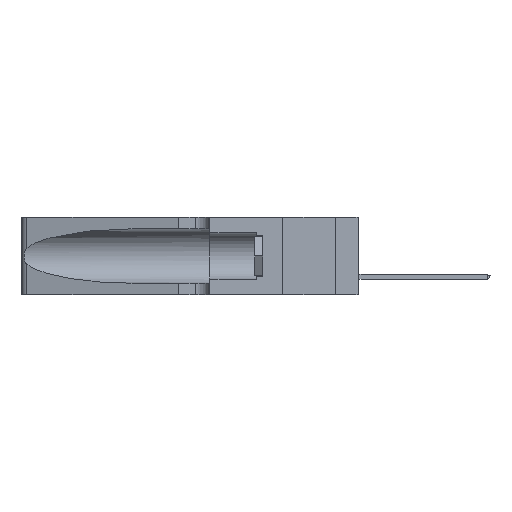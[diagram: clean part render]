
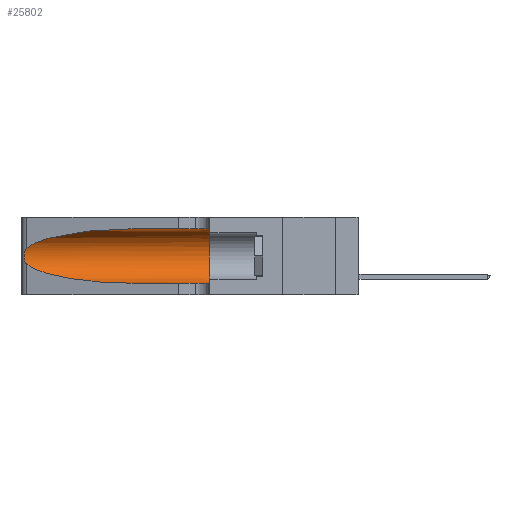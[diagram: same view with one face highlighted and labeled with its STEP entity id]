
A CAD part, left-side view. The second image highlights one B-rep face of the part: STEP entity #25802.
In plain terms, the highlighted cylindrical face has radius 3.308 mm (diameter 6.617 mm), a partial arc.
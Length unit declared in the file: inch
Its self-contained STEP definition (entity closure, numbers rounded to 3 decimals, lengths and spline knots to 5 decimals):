
#329 = CARTESIAN_POINT ( 'NONE',  ( 0.2373, 1.15595, 0.28018 ) ) ;
#466 = CARTESIAN_POINT ( 'NONE',  ( 0.25487, 1.22718, 0.22369 ) ) ;
#646 = B_SPLINE_CURVE_WITH_KNOTS ( 'NONE', 3,
 ( #31144, #28114, #27735, #3886, #34121, #25180, #22039, #28248, #15803, #9945, #12984, #37302, #15932, #9828 ),
 .UNSPECIFIED., .F., .F.,
 ( 4, 2, 2, 2, 2, 2, 4 ),
 ( 0., 0.00027, 0.00053, 0.00107, 0.0016, 0.00187, 0.00214 ),
 .UNSPECIFIED. ) ;
#968 = VERTEX_POINT ( 'NONE', #14451 ) ;
#1594 = EDGE_LOOP ( 'NONE', ( #10180, #10909, #35778, #21880, #19477, #6456 ) ) ;
#3886 = CARTESIAN_POINT ( 'NONE',  ( 0.25787, 1.23484, 0.2124 ) ) ;
#5508 = LINE ( 'NONE', #15511, #12662 ) ;
#5999 = VECTOR ( 'NONE', #31291, 39.37008 ) ;
#6345 = CARTESIAN_POINT ( 'NONE',  ( 0.1305, 0.35, 0.185 ) ) ;
#6393 = CARTESIAN_POINT ( 'NONE',  ( 0.18966, 0.96281, 0.05475 ) ) ;
#6456 = ORIENTED_EDGE ( 'NONE', *, *, #38865, .F. ) ;
#6524 = CARTESIAN_POINT ( 'NONE',  ( 0.1305, 0.72297, 0.05475 ) ) ;
#7935 = DIRECTION ( 'NONE',  ( 0., 0., -1. ) ) ;
#8790 = CARTESIAN_POINT ( 'NONE',  ( 0.25487, 1.22718, 0.14631 ) ) ;
#8874 = EDGE_CURVE ( 'NONE', #18250, #968, #15848, .T. ) ;
#8904 = EDGE_CURVE ( 'NONE', #26192, #28941, #13090, .T. ) ;
#9648 = CARTESIAN_POINT ( 'NONE',  ( 0.2373, 1.15595, 0.08982 ) ) ;
#9828 = CARTESIAN_POINT ( 'NONE',  ( 0.25487, 1.22718, 0.14631 ) ) ;
#9945 = CARTESIAN_POINT ( 'NONE',  ( 0.25856, 1.23593, 0.16098 ) ) ;
#10146 = EDGE_CURVE ( 'NONE', #27516, #968, #16982, .T. ) ;
#10180 = ORIENTED_EDGE ( 'NONE', *, *, #8904, .T. ) ;
#10192 = CARTESIAN_POINT ( 'NONE',  ( 0.25487, 1.22718, 0.22369 ) ) ;
#10909 = ORIENTED_EDGE ( 'NONE', *, *, #31441, .T. ) ;
#11283 = AXIS2_PLACEMENT_3D ( 'NONE', #14446, #35176, #7935 ) ;
#12662 = VECTOR ( 'NONE', #27305, 39.37008 ) ;
#12984 = CARTESIAN_POINT ( 'NONE',  ( 0.25789, 1.23486, 0.15765 ) ) ;
#13090 =( BOUNDED_CURVE ( )  B_SPLINE_CURVE ( 3, ( #21800, #24837, #329, #466 ),
 .UNSPECIFIED., .F., .F. ) 
 B_SPLINE_CURVE_WITH_KNOTS ( ( 4, 4 ),
 ( 1.5708, 2.84003 ),
 .UNSPECIFIED. ) 
 CURVE ( )  GEOMETRIC_REPRESENTATION_ITEM ( )  RATIONAL_B_SPLINE_CURVE ( ( 1., 0.87, 0.87, 1. ) ) 
 REPRESENTATION_ITEM ( '' )  );
#13097 = CARTESIAN_POINT ( 'NONE',  ( 0.1305, 0.72297, 0.31525 ) ) ;
#13252 = CARTESIAN_POINT ( 'NONE',  ( 0.1305, 1.61858, 0.05475 ) ) ;
#14446 = CARTESIAN_POINT ( 'NONE',  ( 0.1305, 1.61858, 0.185 ) ) ;
#14451 = CARTESIAN_POINT ( 'NONE',  ( 0.1305, 0.35, 0.05475 ) ) ;
#14582 = VERTEX_POINT ( 'NONE', #8790 ) ;
#15511 = CARTESIAN_POINT ( 'NONE',  ( 0.1305, 1.61858, 0.31525 ) ) ;
#15620 = CARTESIAN_POINT ( 'NONE',  ( 0.1305, 0.35, 0.31525 ) ) ;
#15743 = AXIS2_PLACEMENT_3D ( 'NONE', #6345, #27483, #36151 ) ;
#15748 = CARTESIAN_POINT ( 'NONE',  ( 0.25487, 1.22718, 0.14631 ) ) ;
#15803 = CARTESIAN_POINT ( 'NONE',  ( 0.26017, 1.23833, 0.17102 ) ) ;
#15848 = CIRCLE ( 'NONE', #15743, 0.13025 ) ;
#15884 = CYLINDRICAL_SURFACE ( 'NONE', #11283, 0.13025 ) ;
#15932 = CARTESIAN_POINT ( 'NONE',  ( 0.25555, 1.22993, 0.14849 ) ) ;
#16982 = LINE ( 'NONE', #13252, #5999 ) ;
#18250 = VERTEX_POINT ( 'NONE', #15620 ) ;
#19477 = ORIENTED_EDGE ( 'NONE', *, *, #8874, .F. ) ;
#21800 = CARTESIAN_POINT ( 'NONE',  ( 0.1305, 0.72297, 0.31525 ) ) ;
#21880 = ORIENTED_EDGE ( 'NONE', *, *, #10146, .T. ) ;
#22039 = CARTESIAN_POINT ( 'NONE',  ( 0.26075, 1.23896, 0.19203 ) ) ;
#24792 = EDGE_CURVE ( 'NONE', #14582, #27516, #26023, .T. ) ;
#24837 = CARTESIAN_POINT ( 'NONE',  ( 0.18966, 0.96281, 0.31525 ) ) ;
#25180 = CARTESIAN_POINT ( 'NONE',  ( 0.26018, 1.23835, 0.19895 ) ) ;
#25802 = ADVANCED_FACE ( 'NONE', ( #34387 ), #15884, .F. ) ;
#26023 =( BOUNDED_CURVE ( )  B_SPLINE_CURVE ( 3, ( #15748, #9648, #6393, #6524 ),
 .UNSPECIFIED., .F., .F. ) 
 B_SPLINE_CURVE_WITH_KNOTS ( ( 4, 4 ),
 ( 3.44316, 4.71239 ),
 .UNSPECIFIED. ) 
 CURVE ( )  GEOMETRIC_REPRESENTATION_ITEM ( )  RATIONAL_B_SPLINE_CURVE ( ( 1., 0.87, 0.87, 1. ) ) 
 REPRESENTATION_ITEM ( '' )  );
#26192 = VERTEX_POINT ( 'NONE', #13097 ) ;
#27305 = DIRECTION ( 'NONE',  ( 0., -1., 0. ) ) ;
#27483 = DIRECTION ( 'NONE',  ( 0., 1., 0. ) ) ;
#27516 = VERTEX_POINT ( 'NONE', #36046 ) ;
#27735 = CARTESIAN_POINT ( 'NONE',  ( 0.25639, 1.23184, 0.21858 ) ) ;
#28114 = CARTESIAN_POINT ( 'NONE',  ( 0.25555, 1.22994, 0.2215 ) ) ;
#28248 = CARTESIAN_POINT ( 'NONE',  ( 0.26075, 1.23896, 0.178 ) ) ;
#28941 = VERTEX_POINT ( 'NONE', #10192 ) ;
#31144 = CARTESIAN_POINT ( 'NONE',  ( 0.25487, 1.22718, 0.22369 ) ) ;
#31291 = DIRECTION ( 'NONE',  ( 0., -1., 0. ) ) ;
#31441 = EDGE_CURVE ( 'NONE', #28941, #14582, #646, .T. ) ;
#34121 = CARTESIAN_POINT ( 'NONE',  ( 0.25854, 1.2359, 0.20912 ) ) ;
#34387 = FACE_OUTER_BOUND ( 'NONE', #1594, .T. ) ;
#35176 = DIRECTION ( 'NONE',  ( 0., -1., 0. ) ) ;
#35778 = ORIENTED_EDGE ( 'NONE', *, *, #24792, .T. ) ;
#36046 = CARTESIAN_POINT ( 'NONE',  ( 0.1305, 0.72297, 0.05475 ) ) ;
#36151 = DIRECTION ( 'NONE',  ( 0., 0., 1. ) ) ;
#37302 = CARTESIAN_POINT ( 'NONE',  ( 0.25639, 1.23186, 0.15144 ) ) ;
#38865 = EDGE_CURVE ( 'NONE', #26192, #18250, #5508, .T. ) ;
